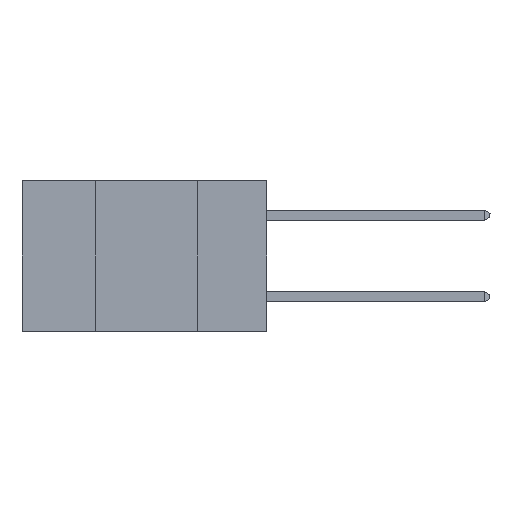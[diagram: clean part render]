
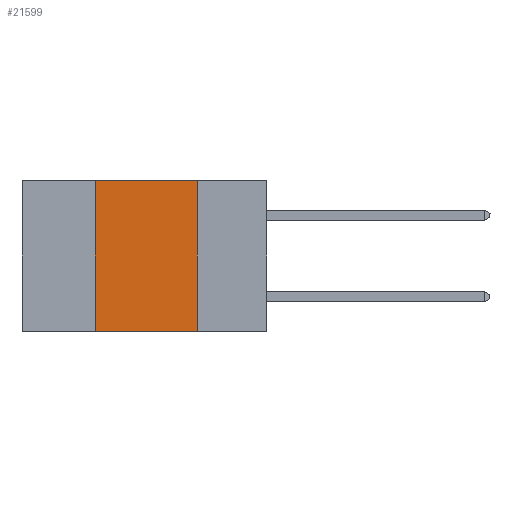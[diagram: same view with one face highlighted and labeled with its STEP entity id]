
A CAD part, left-side view. The second image highlights one B-rep face of the part: STEP entity #21599.
In plain terms, the highlighted planar face has unit normal (-1, 0, 0).
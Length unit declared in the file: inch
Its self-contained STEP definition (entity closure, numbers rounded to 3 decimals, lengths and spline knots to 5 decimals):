
#1874 = DIRECTION ( 'NONE',  ( 1., 0., 0. ) ) ;
#4407 = EDGE_CURVE ( 'NONE', #11733, #23860, #19006, .T. ) ;
#4896 = LINE ( 'NONE', #31258, #22561 ) ;
#5494 = ORIENTED_EDGE ( 'NONE', *, *, #4407, .T. ) ;
#9026 = VECTOR ( 'NONE', #35701, 39.37008 ) ;
#9210 = LINE ( 'NONE', #17394, #31284 ) ;
#9512 = VERTEX_POINT ( 'NONE', #34413 ) ;
#11733 = VERTEX_POINT ( 'NONE', #25586 ) ;
#12183 = EDGE_CURVE ( 'NONE', #11733, #34952, #4896, .T. ) ;
#12571 = ORIENTED_EDGE ( 'NONE', *, *, #34508, .F. ) ;
#13442 = CARTESIAN_POINT ( 'NONE',  ( 0., 0.17, 0. ) ) ;
#14417 = VECTOR ( 'NONE', #19505, 39.37008 ) ;
#15268 = AXIS2_PLACEMENT_3D ( 'NONE', #27285, #1874, #18943 ) ;
#16306 = EDGE_CURVE ( 'NONE', #34952, #9512, #9210, .T. ) ;
#16474 = DIRECTION ( 'NONE',  ( 0., 0., 1. ) ) ;
#17394 = CARTESIAN_POINT ( 'NONE',  ( 0., 0.6, 0. ) ) ;
#18943 = DIRECTION ( 'NONE',  ( 0., 0., -1. ) ) ;
#19006 = LINE ( 'NONE', #32871, #9026 ) ;
#19505 = DIRECTION ( 'NONE',  ( 0., 0., -1. ) ) ;
#21599 = ADVANCED_FACE ( 'NONE', ( #22164 ), #36384, .F. ) ;
#22164 = FACE_OUTER_BOUND ( 'NONE', #26736, .T. ) ;
#22561 = VECTOR ( 'NONE', #16474, 39.37008 ) ;
#22924 = DIRECTION ( 'NONE',  ( 0., -1., 0. ) ) ;
#23860 = VERTEX_POINT ( 'NONE', #31186 ) ;
#25586 = CARTESIAN_POINT ( 'NONE',  ( 0., 0.42, -0.37 ) ) ;
#26736 = EDGE_LOOP ( 'NONE', ( #12571, #28253, #33755, #5494 ) ) ;
#27188 = CARTESIAN_POINT ( 'NONE',  ( 0., 0.42, 0. ) ) ;
#27285 = CARTESIAN_POINT ( 'NONE',  ( 0., 0.6, 0. ) ) ;
#28253 = ORIENTED_EDGE ( 'NONE', *, *, #16306, .F. ) ;
#31186 = CARTESIAN_POINT ( 'NONE',  ( 0., 0.17, -0.37 ) ) ;
#31258 = CARTESIAN_POINT ( 'NONE',  ( 0., 0.42, 0. ) ) ;
#31284 = VECTOR ( 'NONE', #22924, 39.37008 ) ;
#32871 = CARTESIAN_POINT ( 'NONE',  ( 0., 0.6, -0.37 ) ) ;
#33755 = ORIENTED_EDGE ( 'NONE', *, *, #12183, .F. ) ;
#34413 = CARTESIAN_POINT ( 'NONE',  ( 0., 0.17, 0. ) ) ;
#34508 = EDGE_CURVE ( 'NONE', #9512, #23860, #36948, .T. ) ;
#34952 = VERTEX_POINT ( 'NONE', #27188 ) ;
#35701 = DIRECTION ( 'NONE',  ( 0., -1., 0. ) ) ;
#36384 = PLANE ( 'NONE',  #15268 ) ;
#36948 = LINE ( 'NONE', #13442, #14417 ) ;
